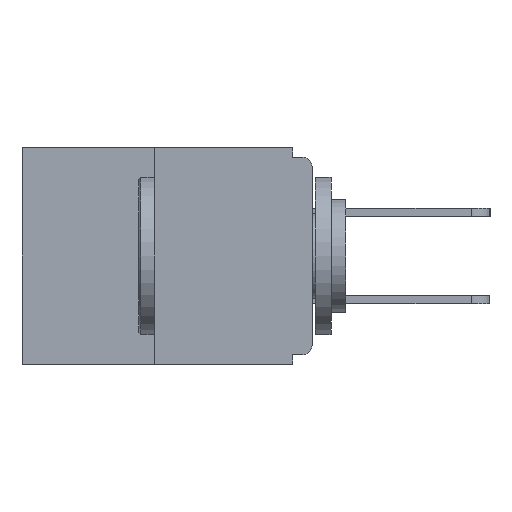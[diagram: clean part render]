
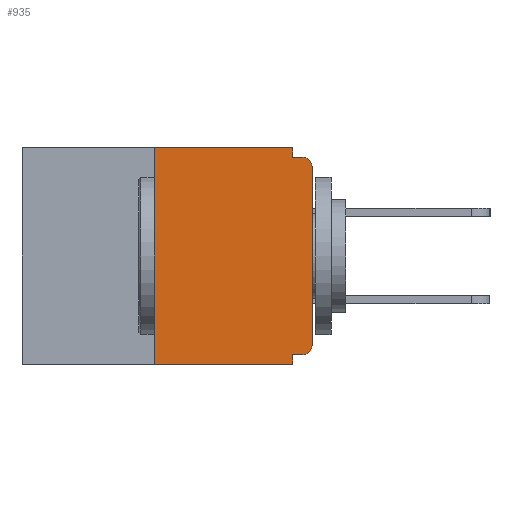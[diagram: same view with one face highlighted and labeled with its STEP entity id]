
A CAD part, left-side view. The second image highlights one B-rep face of the part: STEP entity #935.
In plain terms, the highlighted planar face has unit normal (-1, 0, 0).
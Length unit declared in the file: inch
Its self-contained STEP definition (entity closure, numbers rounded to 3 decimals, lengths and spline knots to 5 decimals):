
#112 = VERTEX_POINT ( 'NONE', #810 ) ;
#143 = DIRECTION ( 'NONE',  ( 0., 0., -1. ) ) ;
#484 = CARTESIAN_POINT ( 'NONE',  ( 0., 0.46, 0. ) ) ;
#515 = VERTEX_POINT ( 'NONE', #9610 ) ;
#810 = CARTESIAN_POINT ( 'NONE',  ( 0., 0., -0.313 ) ) ;
#843 = EDGE_CURVE ( 'NONE', #16759, #1655, #7441, .T. ) ;
#925 = LINE ( 'NONE', #16146, #2725 ) ;
#935 = ADVANCED_FACE ( 'NONE', ( #2790 ), #14559, .F. ) ;
#1290 = CARTESIAN_POINT ( 'NONE',  ( 0., 0., -0.03 ) ) ;
#1475 = AXIS2_PLACEMENT_3D ( 'NONE', #12019, #5473, #13332 ) ;
#1655 = VERTEX_POINT ( 'NONE', #12451 ) ;
#1657 = CARTESIAN_POINT ( 'NONE',  ( 0., 0.031, 0. ) ) ;
#1771 = VECTOR ( 'NONE', #5447, 39.37008 ) ;
#2112 = CARTESIAN_POINT ( 'NONE',  ( 0., 0.46, -0.343 ) ) ;
#2725 = VECTOR ( 'NONE', #14682, 39.37008 ) ;
#2790 = FACE_OUTER_BOUND ( 'NONE', #14934, .T. ) ;
#2946 = EDGE_CURVE ( 'NONE', #14926, #515, #5980, .T. ) ;
#3852 = ORIENTED_EDGE ( 'NONE', *, *, #10347, .F. ) ;
#3981 = EDGE_CURVE ( 'NONE', #11144, #112, #9960, .T. ) ;
#4035 = EDGE_CURVE ( 'NONE', #15750, #9997, #15885, .T. ) ;
#4416 = CARTESIAN_POINT ( 'NONE',  ( 0., 0.031, -0.343 ) ) ;
#4504 = VECTOR ( 'NONE', #7456, 39.37008 ) ;
#4727 = CARTESIAN_POINT ( 'NONE',  ( 0., 0.25, -0.343 ) ) ;
#4808 = ORIENTED_EDGE ( 'NONE', *, *, #3981, .T. ) ;
#4950 = EDGE_CURVE ( 'NONE', #11144, #15750, #8513, .T. ) ;
#5313 = LINE ( 'NONE', #10044, #4504 ) ;
#5447 = DIRECTION ( 'NONE',  ( 0., 0., 1. ) ) ;
#5467 = ORIENTED_EDGE ( 'NONE', *, *, #12777, .F. ) ;
#5473 = DIRECTION ( 'NONE',  ( -1., 0., 0. ) ) ;
#5652 = DIRECTION ( 'NONE',  ( 0., 0., -1. ) ) ;
#5740 = DIRECTION ( 'NONE',  ( -1., 0., 0. ) ) ;
#5980 = CIRCLE ( 'NONE', #14649, 0.015 ) ;
#6076 = VECTOR ( 'NONE', #8785, 39.37008 ) ;
#6272 = VERTEX_POINT ( 'NONE', #4727 ) ;
#6494 = CARTESIAN_POINT ( 'NONE',  ( 0., 0.031, -0.328 ) ) ;
#7441 = LINE ( 'NONE', #1657, #14802 ) ;
#7456 = DIRECTION ( 'NONE',  ( 0., -1., 0. ) ) ;
#7671 = ORIENTED_EDGE ( 'NONE', *, *, #843, .F. ) ;
#8143 = LINE ( 'NONE', #2112, #8565 ) ;
#8186 = EDGE_CURVE ( 'NONE', #11975, #16759, #925, .T. ) ;
#8282 = ORIENTED_EDGE ( 'NONE', *, *, #9757, .T. ) ;
#8328 = CARTESIAN_POINT ( 'NONE',  ( 0., 0.015, -0.03 ) ) ;
#8513 = LINE ( 'NONE', #12820, #6076 ) ;
#8565 = VECTOR ( 'NONE', #16145, 39.37008 ) ;
#8785 = DIRECTION ( 'NONE',  ( 0., 1., 0. ) ) ;
#8786 = ORIENTED_EDGE ( 'NONE', *, *, #4950, .F. ) ;
#9528 = CARTESIAN_POINT ( 'NONE',  ( 0., 0., 0. ) ) ;
#9553 = DIRECTION ( 'NONE',  ( 1., 0., 0. ) ) ;
#9610 = CARTESIAN_POINT ( 'NONE',  ( 0., 0.015, -0.015 ) ) ;
#9691 = DIRECTION ( 'NONE',  ( 0., 0., -1. ) ) ;
#9757 = EDGE_CURVE ( 'NONE', #6272, #9997, #8143, .T. ) ;
#9772 = VECTOR ( 'NONE', #143, 39.37008 ) ;
#9958 = ORIENTED_EDGE ( 'NONE', *, *, #11149, .T. ) ;
#9960 = CIRCLE ( 'NONE', #1475, 0.015 ) ;
#9997 = VERTEX_POINT ( 'NONE', #4416 ) ;
#10044 = CARTESIAN_POINT ( 'NONE',  ( 0., 0., -0.015 ) ) ;
#10266 = LINE ( 'NONE', #9528, #10899 ) ;
#10347 = EDGE_CURVE ( 'NONE', #6272, #11975, #16002, .T. ) ;
#10596 = CARTESIAN_POINT ( 'NONE',  ( 0., 0.031, -0.343 ) ) ;
#10786 = CARTESIAN_POINT ( 'NONE',  ( 0., 0.25, 0. ) ) ;
#10834 = DIRECTION ( 'NONE',  ( 0., 0., -1. ) ) ;
#10899 = VECTOR ( 'NONE', #16165, 39.37008 ) ;
#10998 = CARTESIAN_POINT ( 'NONE',  ( 0., 0.031, 0. ) ) ;
#11144 = VERTEX_POINT ( 'NONE', #13485 ) ;
#11149 = EDGE_CURVE ( 'NONE', #112, #14926, #10266, .T. ) ;
#11322 = AXIS2_PLACEMENT_3D ( 'NONE', #484, #9553, #10834 ) ;
#11975 = VERTEX_POINT ( 'NONE', #16084 ) ;
#12019 = CARTESIAN_POINT ( 'NONE',  ( 0., 0.015, -0.313 ) ) ;
#12451 = CARTESIAN_POINT ( 'NONE',  ( 0., 0.031, -0.015 ) ) ;
#12777 = EDGE_CURVE ( 'NONE', #1655, #515, #5313, .T. ) ;
#12820 = CARTESIAN_POINT ( 'NONE',  ( 0., 0., -0.328 ) ) ;
#13332 = DIRECTION ( 'NONE',  ( 0., 0., -1. ) ) ;
#13485 = CARTESIAN_POINT ( 'NONE',  ( 0., 0.015, -0.328 ) ) ;
#14338 = ORIENTED_EDGE ( 'NONE', *, *, #4035, .F. ) ;
#14559 = PLANE ( 'NONE',  #11322 ) ;
#14649 = AXIS2_PLACEMENT_3D ( 'NONE', #8328, #5740, #9691 ) ;
#14682 = DIRECTION ( 'NONE',  ( 0., -1., 0. ) ) ;
#14802 = VECTOR ( 'NONE', #5652, 39.37008 ) ;
#14926 = VERTEX_POINT ( 'NONE', #1290 ) ;
#14934 = EDGE_LOOP ( 'NONE', ( #15208, #3852, #8282, #14338, #8786, #4808, #9958, #16605, #5467, #7671 ) ) ;
#15208 = ORIENTED_EDGE ( 'NONE', *, *, #8186, .F. ) ;
#15750 = VERTEX_POINT ( 'NONE', #6494 ) ;
#15885 = LINE ( 'NONE', #10596, #9772 ) ;
#16002 = LINE ( 'NONE', #10786, #1771 ) ;
#16084 = CARTESIAN_POINT ( 'NONE',  ( 0., 0.25, 0. ) ) ;
#16145 = DIRECTION ( 'NONE',  ( 0., -1., 0. ) ) ;
#16146 = CARTESIAN_POINT ( 'NONE',  ( 0., 0.46, 0. ) ) ;
#16165 = DIRECTION ( 'NONE',  ( 0., 0., 1. ) ) ;
#16605 = ORIENTED_EDGE ( 'NONE', *, *, #2946, .T. ) ;
#16759 = VERTEX_POINT ( 'NONE', #10998 ) ;
